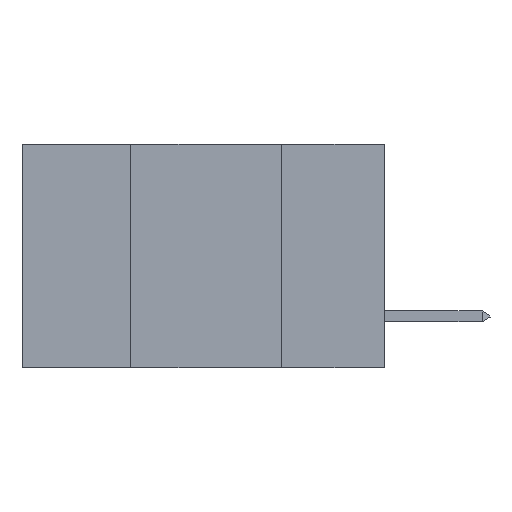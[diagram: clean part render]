
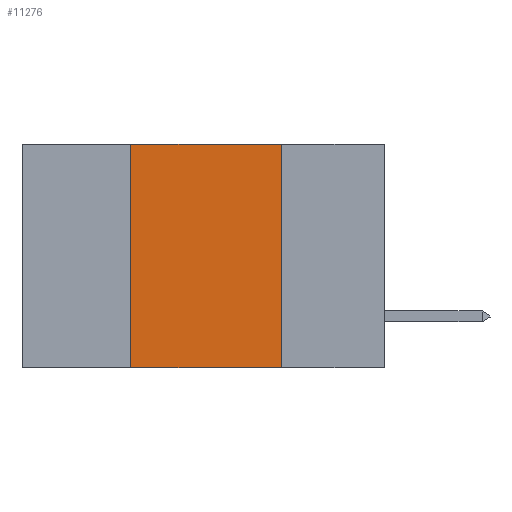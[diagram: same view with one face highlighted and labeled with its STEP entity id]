
A CAD part, left-side view. The second image highlights one B-rep face of the part: STEP entity #11276.
In plain terms, the highlighted planar face has unit normal (-1, 0, 0).
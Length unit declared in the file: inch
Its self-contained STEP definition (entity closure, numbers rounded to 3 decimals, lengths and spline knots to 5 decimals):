
#587 = DIRECTION ( 'NONE',  ( 0., 0., -1. ) ) ;
#672 = VERTEX_POINT ( 'NONE', #5372 ) ;
#1260 = VERTEX_POINT ( 'NONE', #8646 ) ;
#1507 = ORIENTED_EDGE ( 'NONE', *, *, #7682, .F. ) ;
#1578 = VECTOR ( 'NONE', #12590, 39.37008 ) ;
#1657 = VECTOR ( 'NONE', #10228, 39.37008 ) ;
#1958 = CARTESIAN_POINT ( 'NONE',  ( 0., 0.17, 0. ) ) ;
#2237 = VECTOR ( 'NONE', #6549, 39.37008 ) ;
#2697 = CARTESIAN_POINT ( 'NONE',  ( 0., 0.17, -0.37 ) ) ;
#3418 = ORIENTED_EDGE ( 'NONE', *, *, #13164, .T. ) ;
#3686 = CARTESIAN_POINT ( 'NONE',  ( 0., 0.42, 0. ) ) ;
#4327 = EDGE_LOOP ( 'NONE', ( #9080, #8430, #1507, #3418 ) ) ;
#4620 = DIRECTION ( 'NONE',  ( 1., 0., 0. ) ) ;
#4691 = CARTESIAN_POINT ( 'NONE',  ( 0., 0.17, 0. ) ) ;
#5372 = CARTESIAN_POINT ( 'NONE',  ( 0., 0.42, 0. ) ) ;
#5420 = VERTEX_POINT ( 'NONE', #4691 ) ;
#5748 = CARTESIAN_POINT ( 'NONE',  ( 0., 0.6, 0. ) ) ;
#6549 = DIRECTION ( 'NONE',  ( 0., -1., 0. ) ) ;
#6728 = CARTESIAN_POINT ( 'NONE',  ( 0., 0.6, 0. ) ) ;
#7248 = VERTEX_POINT ( 'NONE', #2697 ) ;
#7682 = EDGE_CURVE ( 'NONE', #1260, #672, #8761, .T. ) ;
#8152 = FACE_OUTER_BOUND ( 'NONE', #4327, .T. ) ;
#8283 = AXIS2_PLACEMENT_3D ( 'NONE', #6728, #4620, #587 ) ;
#8430 = ORIENTED_EDGE ( 'NONE', *, *, #11188, .F. ) ;
#8646 = CARTESIAN_POINT ( 'NONE',  ( 0., 0.42, -0.37 ) ) ;
#8685 = LINE ( 'NONE', #1958, #1657 ) ;
#8761 = LINE ( 'NONE', #3686, #9088 ) ;
#9080 = ORIENTED_EDGE ( 'NONE', *, *, #9732, .F. ) ;
#9088 = VECTOR ( 'NONE', #10876, 39.37008 ) ;
#9374 = CARTESIAN_POINT ( 'NONE',  ( 0., 0.6, -0.37 ) ) ;
#9485 = LINE ( 'NONE', #5748, #2237 ) ;
#9732 = EDGE_CURVE ( 'NONE', #5420, #7248, #8685, .T. ) ;
#10228 = DIRECTION ( 'NONE',  ( 0., 0., -1. ) ) ;
#10876 = DIRECTION ( 'NONE',  ( 0., 0., 1. ) ) ;
#11188 = EDGE_CURVE ( 'NONE', #672, #5420, #9485, .T. ) ;
#11276 = ADVANCED_FACE ( 'NONE', ( #8152 ), #12909, .F. ) ;
#11869 = LINE ( 'NONE', #9374, #1578 ) ;
#12590 = DIRECTION ( 'NONE',  ( 0., -1., 0. ) ) ;
#12909 = PLANE ( 'NONE',  #8283 ) ;
#13164 = EDGE_CURVE ( 'NONE', #1260, #7248, #11869, .T. ) ;
